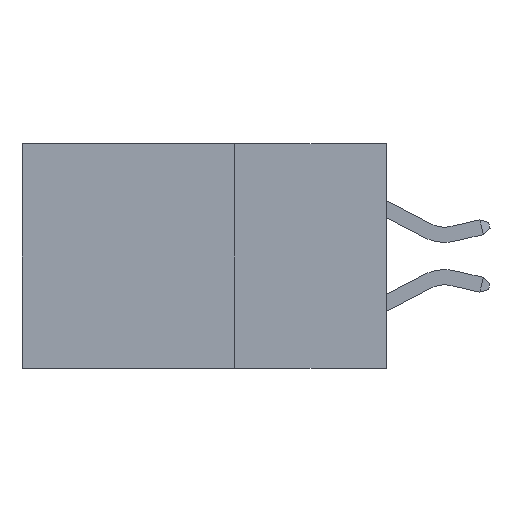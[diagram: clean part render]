
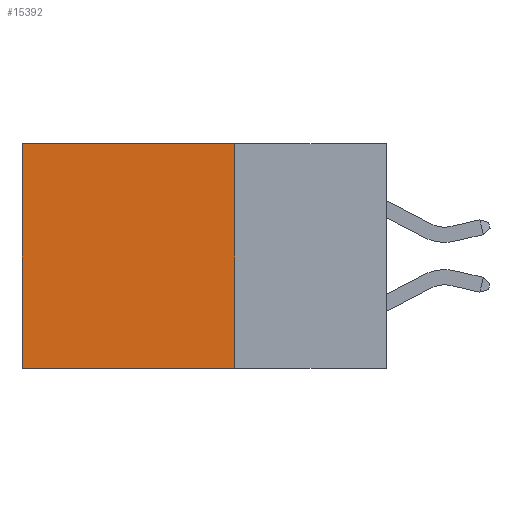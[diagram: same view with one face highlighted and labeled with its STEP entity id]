
A CAD part, left-side view. The second image highlights one B-rep face of the part: STEP entity #15392.
In plain terms, the highlighted planar face has unit normal (-1, 0, 0).
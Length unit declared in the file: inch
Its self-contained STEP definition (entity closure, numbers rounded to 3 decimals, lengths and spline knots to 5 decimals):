
#560 = FACE_OUTER_BOUND ( 'NONE', #7479, .T. ) ;
#1057 = DIRECTION ( 'NONE',  ( 0., 1., 0. ) ) ;
#2099 = LINE ( 'NONE', #13457, #10971 ) ;
#2485 = CARTESIAN_POINT ( 'NONE',  ( 0.2615, 0.25, 0. ) ) ;
#3186 = LINE ( 'NONE', #2485, #11443 ) ;
#3526 = EDGE_CURVE ( 'NONE', #5409, #10551, #2099, .T. ) ;
#3611 = AXIS2_PLACEMENT_3D ( 'NONE', #10763, #17723, #7375 ) ;
#5232 = CARTESIAN_POINT ( 'NONE',  ( 0.2615, 0.25, -0.37 ) ) ;
#5409 = VERTEX_POINT ( 'NONE', #11050 ) ;
#6001 = ORIENTED_EDGE ( 'NONE', *, *, #18725, .F. ) ;
#6673 = CARTESIAN_POINT ( 'NONE',  ( 0.2615, 0.25, -0.37 ) ) ;
#7375 = DIRECTION ( 'NONE',  ( 0., 0., -1. ) ) ;
#7479 = EDGE_LOOP ( 'NONE', ( #9686, #6001, #12474, #12293 ) ) ;
#7680 = VECTOR ( 'NONE', #1057, 39.37008 ) ;
#8036 = VERTEX_POINT ( 'NONE', #20835 ) ;
#8240 = CARTESIAN_POINT ( 'NONE',  ( 0.2615, 0.25, -0.37 ) ) ;
#8418 = DIRECTION ( 'NONE',  ( 0., 0., -1. ) ) ;
#8781 = VERTEX_POINT ( 'NONE', #5232 ) ;
#9686 = ORIENTED_EDGE ( 'NONE', *, *, #3526, .T. ) ;
#10551 = VERTEX_POINT ( 'NONE', #14801 ) ;
#10763 = CARTESIAN_POINT ( 'NONE',  ( 0.2615, 0.25, -0.37 ) ) ;
#10971 = VECTOR ( 'NONE', #13583, 39.37008 ) ;
#11050 = CARTESIAN_POINT ( 'NONE',  ( 0.2615, 0.6, 0. ) ) ;
#11106 = LINE ( 'NONE', #6673, #19793 ) ;
#11443 = VECTOR ( 'NONE', #16513, 39.37008 ) ;
#12293 = ORIENTED_EDGE ( 'NONE', *, *, #20476, .T. ) ;
#12474 = ORIENTED_EDGE ( 'NONE', *, *, #22036, .F. ) ;
#13457 = CARTESIAN_POINT ( 'NONE',  ( 0.2615, 0.6, -0.37 ) ) ;
#13583 = DIRECTION ( 'NONE',  ( 0., 0., -1. ) ) ;
#14284 = PLANE ( 'NONE',  #3611 ) ;
#14801 = CARTESIAN_POINT ( 'NONE',  ( 0.2615, 0.6, -0.37 ) ) ;
#15392 = ADVANCED_FACE ( 'NONE', ( #560 ), #14284, .F. ) ;
#16513 = DIRECTION ( 'NONE',  ( 0., 1., 0. ) ) ;
#17723 = DIRECTION ( 'NONE',  ( 1., 0., 0. ) ) ;
#17963 = LINE ( 'NONE', #8240, #7680 ) ;
#18725 = EDGE_CURVE ( 'NONE', #8781, #10551, #17963, .T. ) ;
#19793 = VECTOR ( 'NONE', #8418, 39.37008 ) ;
#20476 = EDGE_CURVE ( 'NONE', #8036, #5409, #3186, .T. ) ;
#20835 = CARTESIAN_POINT ( 'NONE',  ( 0.2615, 0.25, 0. ) ) ;
#22036 = EDGE_CURVE ( 'NONE', #8036, #8781, #11106, .T. ) ;
